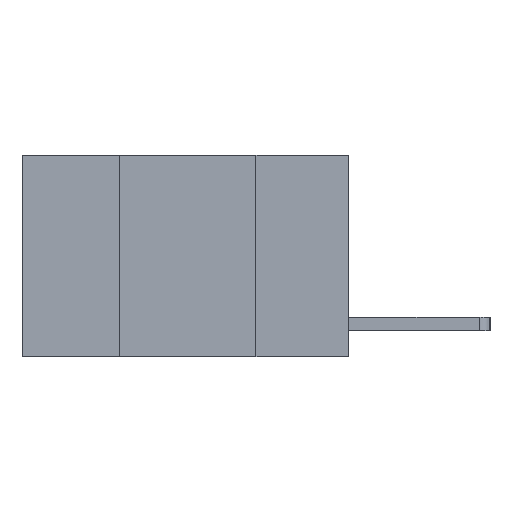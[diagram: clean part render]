
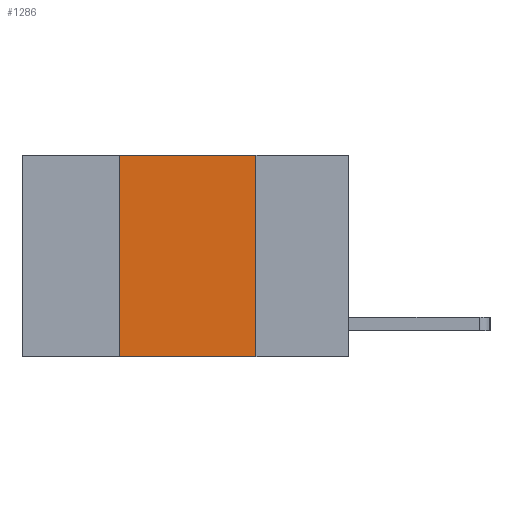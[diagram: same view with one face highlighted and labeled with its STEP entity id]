
A CAD part, left-side view. The second image highlights one B-rep face of the part: STEP entity #1286.
In plain terms, the highlighted planar face has unit normal (-1, 0, 0).
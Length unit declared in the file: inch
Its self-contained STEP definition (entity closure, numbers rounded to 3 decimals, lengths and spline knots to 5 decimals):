
#67 = EDGE_CURVE ( 'NONE', #8085, #4810, #4225, .T. ) ;
#246 = EDGE_CURVE ( 'NONE', #4720, #4810, #3473, .T. ) ;
#909 = AXIS2_PLACEMENT_3D ( 'NONE', #4687, #2297, #4735 ) ;
#982 = DIRECTION ( 'NONE',  ( 0., 0., 1. ) ) ;
#1189 = CARTESIAN_POINT ( 'NONE',  ( 0., 0.42, -0.37 ) ) ;
#1286 = ADVANCED_FACE ( 'NONE', ( #3062 ), #7708, .F. ) ;
#2200 = ORIENTED_EDGE ( 'NONE', *, *, #3980, .F. ) ;
#2297 = DIRECTION ( 'NONE',  ( 1., 0., 0. ) ) ;
#2856 = EDGE_LOOP ( 'NONE', ( #3431, #2200, #4623, #3877 ) ) ;
#3033 = CARTESIAN_POINT ( 'NONE',  ( 0., 0.42, 0. ) ) ;
#3062 = FACE_OUTER_BOUND ( 'NONE', #2856, .T. ) ;
#3172 = DIRECTION ( 'NONE',  ( 0., -1., 0. ) ) ;
#3353 = VECTOR ( 'NONE', #3172, 39.37008 ) ;
#3431 = ORIENTED_EDGE ( 'NONE', *, *, #67, .F. ) ;
#3473 = LINE ( 'NONE', #8656, #3353 ) ;
#3483 = VECTOR ( 'NONE', #8030, 39.37008 ) ;
#3545 = EDGE_CURVE ( 'NONE', #4720, #7898, #5271, .T. ) ;
#3849 = LINE ( 'NONE', #6264, #3483 ) ;
#3877 = ORIENTED_EDGE ( 'NONE', *, *, #246, .T. ) ;
#3980 = EDGE_CURVE ( 'NONE', #7898, #8085, #3849, .T. ) ;
#4225 = LINE ( 'NONE', #5163, #4402 ) ;
#4402 = VECTOR ( 'NONE', #7661, 39.37008 ) ;
#4623 = ORIENTED_EDGE ( 'NONE', *, *, #3545, .F. ) ;
#4687 = CARTESIAN_POINT ( 'NONE',  ( 0., 0.6, 0. ) ) ;
#4720 = VERTEX_POINT ( 'NONE', #1189 ) ;
#4731 = CARTESIAN_POINT ( 'NONE',  ( 0., 0.17, 0. ) ) ;
#4735 = DIRECTION ( 'NONE',  ( 0., 0., -1. ) ) ;
#4810 = VERTEX_POINT ( 'NONE', #5451 ) ;
#5163 = CARTESIAN_POINT ( 'NONE',  ( 0., 0.17, 0. ) ) ;
#5176 = CARTESIAN_POINT ( 'NONE',  ( 0., 0.42, 0. ) ) ;
#5252 = VECTOR ( 'NONE', #982, 39.37008 ) ;
#5271 = LINE ( 'NONE', #5176, #5252 ) ;
#5451 = CARTESIAN_POINT ( 'NONE',  ( 0., 0.17, -0.37 ) ) ;
#6264 = CARTESIAN_POINT ( 'NONE',  ( 0., 0.6, 0. ) ) ;
#7661 = DIRECTION ( 'NONE',  ( 0., 0., -1. ) ) ;
#7708 = PLANE ( 'NONE',  #909 ) ;
#7898 = VERTEX_POINT ( 'NONE', #3033 ) ;
#8030 = DIRECTION ( 'NONE',  ( 0., -1., 0. ) ) ;
#8085 = VERTEX_POINT ( 'NONE', #4731 ) ;
#8656 = CARTESIAN_POINT ( 'NONE',  ( 0., 0.6, -0.37 ) ) ;
